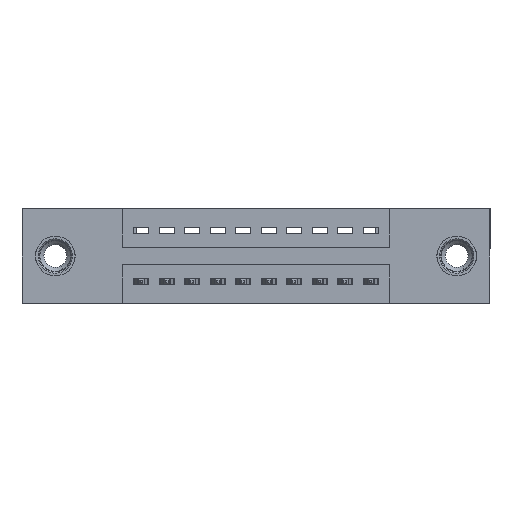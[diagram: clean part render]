
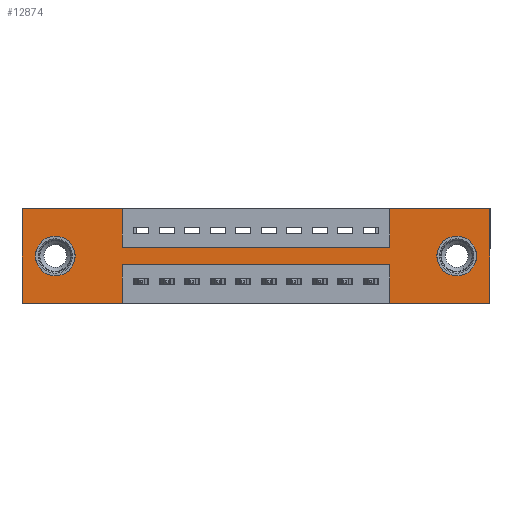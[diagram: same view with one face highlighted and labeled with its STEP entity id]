
A CAD part, front view. The second image highlights one B-rep face of the part: STEP entity #12874.
In plain terms, the highlighted planar face has unit normal (0, -1, 0).
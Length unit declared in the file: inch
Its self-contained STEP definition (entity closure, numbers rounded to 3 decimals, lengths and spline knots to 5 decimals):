
#21 = CARTESIAN_POINT ( 'NONE',  ( 0.3925, 0., -0.37 ) ) ;
#254 = EDGE_CURVE ( 'NONE', #4813, #13213, #10833, .T. ) ;
#297 = CARTESIAN_POINT ( 'NONE',  ( 1.835, 0., -0.37 ) ) ;
#329 = EDGE_CURVE ( 'NONE', #13062, #12910, #3905, .T. ) ;
#353 = CARTESIAN_POINT ( 'NONE',  ( 1.4425, 0., 0. ) ) ;
#485 = FACE_OUTER_BOUND ( 'NONE', #8280, .T. ) ;
#573 = ORIENTED_EDGE ( 'NONE', *, *, #7444, .F. ) ;
#635 = LINE ( 'NONE', #4767, #5573 ) ;
#639 = EDGE_LOOP ( 'NONE', ( #13489, #12977 ) ) ;
#645 = FACE_BOUND ( 'NONE', #639, .T. ) ;
#825 = LINE ( 'NONE', #1271, #7151 ) ;
#924 = VECTOR ( 'NONE', #7887, 39.37008 ) ;
#990 = EDGE_CURVE ( 'NONE', #11762, #13683, #10135, .T. ) ;
#1068 = DIRECTION ( 'NONE',  ( 0., 0., 1. ) ) ;
#1110 = VERTEX_POINT ( 'NONE', #7105 ) ;
#1271 = CARTESIAN_POINT ( 'NONE',  ( 0.3925, 0., 0. ) ) ;
#1292 = ORIENTED_EDGE ( 'NONE', *, *, #13262, .F. ) ;
#1466 = LINE ( 'NONE', #4617, #9600 ) ;
#1613 = CIRCLE ( 'NONE', #13138, 0.078 ) ;
#1667 = DIRECTION ( 'NONE',  ( 0., 1., 0. ) ) ;
#1796 = DIRECTION ( 'NONE',  ( 0., 0., -1. ) ) ;
#1991 = LINE ( 'NONE', #3376, #7304 ) ;
#2018 = EDGE_CURVE ( 'NONE', #13213, #4813, #1613, .T. ) ;
#2021 = DIRECTION ( 'NONE',  ( -1., 0., 0. ) ) ;
#2097 = EDGE_LOOP ( 'NONE', ( #10883, #4486 ) ) ;
#2165 = CARTESIAN_POINT ( 'NONE',  ( 1.4425, 0., -0.15 ) ) ;
#2184 = VECTOR ( 'NONE', #11891, 39.37008 ) ;
#2404 = DIRECTION ( 'NONE',  ( 0., 0., -1. ) ) ;
#2569 = ORIENTED_EDGE ( 'NONE', *, *, #990, .F. ) ;
#2615 = ORIENTED_EDGE ( 'NONE', *, *, #13657, .F. ) ;
#2635 = EDGE_CURVE ( 'NONE', #13719, #9156, #3951, .T. ) ;
#2650 = ORIENTED_EDGE ( 'NONE', *, *, #5373, .F. ) ;
#2685 = VECTOR ( 'NONE', #10183, 39.37008 ) ;
#2769 = CARTESIAN_POINT ( 'NONE',  ( 0., 0., -0.37 ) ) ;
#3183 = ORIENTED_EDGE ( 'NONE', *, *, #4160, .F. ) ;
#3193 = CARTESIAN_POINT ( 'NONE',  ( 0.13, 0., -0.185 ) ) ;
#3329 = EDGE_CURVE ( 'NONE', #9156, #13719, #5635, .T. ) ;
#3376 = CARTESIAN_POINT ( 'NONE',  ( 0.3925, 0., -0.22 ) ) ;
#3476 = DIRECTION ( 'NONE',  ( 1., 0., 0. ) ) ;
#3497 = ORIENTED_EDGE ( 'NONE', *, *, #5838, .F. ) ;
#3560 = VECTOR ( 'NONE', #13207, 39.37008 ) ;
#3574 = PLANE ( 'NONE',  #7757 ) ;
#3626 = VERTEX_POINT ( 'NONE', #6912 ) ;
#3708 = CARTESIAN_POINT ( 'NONE',  ( 0., 0., 0. ) ) ;
#3786 = DIRECTION ( 'NONE',  ( 0., 0., 1. ) ) ;
#3905 = LINE ( 'NONE', #11838, #9671 ) ;
#3951 = CIRCLE ( 'NONE', #12608, 0.078 ) ;
#3990 = CARTESIAN_POINT ( 'NONE',  ( 1.705, 0., -0.185 ) ) ;
#4160 = EDGE_CURVE ( 'NONE', #10180, #9082, #10006, .T. ) ;
#4393 = VERTEX_POINT ( 'NONE', #11444 ) ;
#4460 = ORIENTED_EDGE ( 'NONE', *, *, #5214, .F. ) ;
#4486 = ORIENTED_EDGE ( 'NONE', *, *, #2018, .T. ) ;
#4598 = CARTESIAN_POINT ( 'NONE',  ( 0.3925, 0., -0.37 ) ) ;
#4617 = CARTESIAN_POINT ( 'NONE',  ( 0., 0., 0. ) ) ;
#4648 = AXIS2_PLACEMENT_3D ( 'NONE', #3990, #7301, #10411 ) ;
#4767 = CARTESIAN_POINT ( 'NONE',  ( 0.3925, 0., -0.15 ) ) ;
#4813 = VERTEX_POINT ( 'NONE', #13123 ) ;
#5049 = DIRECTION ( 'NONE',  ( 0., 0., -1. ) ) ;
#5167 = CARTESIAN_POINT ( 'NONE',  ( 0., 0., 0. ) ) ;
#5214 = EDGE_CURVE ( 'NONE', #1110, #4393, #5613, .T. ) ;
#5373 = EDGE_CURVE ( 'NONE', #8755, #3626, #825, .T. ) ;
#5573 = VECTOR ( 'NONE', #11358, 39.37008 ) ;
#5613 = LINE ( 'NONE', #5167, #3560 ) ;
#5635 = CIRCLE ( 'NONE', #4648, 0.078 ) ;
#5718 = DIRECTION ( 'NONE',  ( 0., -1., 0. ) ) ;
#5820 = AXIS2_PLACEMENT_3D ( 'NONE', #11392, #1667, #3786 ) ;
#5838 = EDGE_CURVE ( 'NONE', #9082, #1110, #10962, .T. ) ;
#6062 = VECTOR ( 'NONE', #2021, 39.37008 ) ;
#6241 = CARTESIAN_POINT ( 'NONE',  ( 1.705, 0., -0.107 ) ) ;
#6496 = DIRECTION ( 'NONE',  ( 0., 1., 0. ) ) ;
#6734 = CARTESIAN_POINT ( 'NONE',  ( 1.705, 0., -0.185 ) ) ;
#6805 = ORIENTED_EDGE ( 'NONE', *, *, #8927, .F. ) ;
#6809 = EDGE_CURVE ( 'NONE', #9452, #13062, #1466, .T. ) ;
#6892 = CARTESIAN_POINT ( 'NONE',  ( 1.705, 0., -0.263 ) ) ;
#6912 = CARTESIAN_POINT ( 'NONE',  ( 0.3925, 0., -0.15 ) ) ;
#7029 = DIRECTION ( 'NONE',  ( 0., 0., -1. ) ) ;
#7105 = CARTESIAN_POINT ( 'NONE',  ( 0., 0., -0.37 ) ) ;
#7151 = VECTOR ( 'NONE', #1796, 39.37008 ) ;
#7256 = CARTESIAN_POINT ( 'NONE',  ( 0.3925, 0., -0.22 ) ) ;
#7301 = DIRECTION ( 'NONE',  ( 0., 1., 0. ) ) ;
#7304 = VECTOR ( 'NONE', #12032, 39.37008 ) ;
#7444 = EDGE_CURVE ( 'NONE', #12161, #9452, #13274, .T. ) ;
#7558 = DIRECTION ( 'NONE',  ( 0., 0., 1. ) ) ;
#7757 = AXIS2_PLACEMENT_3D ( 'NONE', #7921, #5718, #13106 ) ;
#7887 = DIRECTION ( 'NONE',  ( 0., 0., 1. ) ) ;
#7921 = CARTESIAN_POINT ( 'NONE',  ( 0., 0., -0.37 ) ) ;
#8280 = EDGE_LOOP ( 'NONE', ( #3183, #1292, #2569, #6805, #12929, #10810, #573, #2615, #2650, #13267, #4460, #3497 ) ) ;
#8353 = CARTESIAN_POINT ( 'NONE',  ( 1.4425, 0., 0. ) ) ;
#8510 = CARTESIAN_POINT ( 'NONE',  ( 0.13, 0., -0.263 ) ) ;
#8755 = VERTEX_POINT ( 'NONE', #13372 ) ;
#8927 = EDGE_CURVE ( 'NONE', #12910, #11762, #11769, .T. ) ;
#8985 = FACE_BOUND ( 'NONE', #2097, .T. ) ;
#9082 = VERTEX_POINT ( 'NONE', #21 ) ;
#9156 = VERTEX_POINT ( 'NONE', #6892 ) ;
#9215 = VECTOR ( 'NONE', #2404, 39.37008 ) ;
#9452 = VERTEX_POINT ( 'NONE', #8353 ) ;
#9600 = VECTOR ( 'NONE', #3476, 39.37008 ) ;
#9671 = VECTOR ( 'NONE', #5049, 39.37008 ) ;
#10006 = LINE ( 'NONE', #4598, #9215 ) ;
#10135 = LINE ( 'NONE', #11844, #13017 ) ;
#10180 = VERTEX_POINT ( 'NONE', #7256 ) ;
#10183 = DIRECTION ( 'NONE',  ( 1., 0., 0. ) ) ;
#10411 = DIRECTION ( 'NONE',  ( 0., 0., -1. ) ) ;
#10810 = ORIENTED_EDGE ( 'NONE', *, *, #6809, .F. ) ;
#10833 = CIRCLE ( 'NONE', #5820, 0.078 ) ;
#10883 = ORIENTED_EDGE ( 'NONE', *, *, #254, .T. ) ;
#10906 = CARTESIAN_POINT ( 'NONE',  ( 1.4425, 0., -0.37 ) ) ;
#10962 = LINE ( 'NONE', #2769, #2184 ) ;
#11271 = CARTESIAN_POINT ( 'NONE',  ( 1.835, 0., 0. ) ) ;
#11358 = DIRECTION ( 'NONE',  ( 1., 0., 0. ) ) ;
#11392 = CARTESIAN_POINT ( 'NONE',  ( 0.13, 0., -0.185 ) ) ;
#11444 = CARTESIAN_POINT ( 'NONE',  ( 0., 0., 0. ) ) ;
#11762 = VERTEX_POINT ( 'NONE', #10906 ) ;
#11769 = LINE ( 'NONE', #12950, #6062 ) ;
#11838 = CARTESIAN_POINT ( 'NONE',  ( 1.835, 0., 0. ) ) ;
#11844 = CARTESIAN_POINT ( 'NONE',  ( 1.4425, 0., -0.37 ) ) ;
#11891 = DIRECTION ( 'NONE',  ( -1., 0., 0. ) ) ;
#12032 = DIRECTION ( 'NONE',  ( -1., 0., 0. ) ) ;
#12161 = VERTEX_POINT ( 'NONE', #2165 ) ;
#12323 = DIRECTION ( 'NONE',  ( 0., 1., 0. ) ) ;
#12608 = AXIS2_PLACEMENT_3D ( 'NONE', #6734, #12323, #7029 ) ;
#12673 = LINE ( 'NONE', #3708, #2685 ) ;
#12874 = ADVANCED_FACE ( 'NONE', ( #645, #8985, #485 ), #3574, .T. ) ;
#12910 = VERTEX_POINT ( 'NONE', #297 ) ;
#12929 = ORIENTED_EDGE ( 'NONE', *, *, #329, .F. ) ;
#12950 = CARTESIAN_POINT ( 'NONE',  ( 0., 0., -0.37 ) ) ;
#12977 = ORIENTED_EDGE ( 'NONE', *, *, #3329, .T. ) ;
#13001 = EDGE_CURVE ( 'NONE', #4393, #8755, #12673, .T. ) ;
#13017 = VECTOR ( 'NONE', #7558, 39.37008 ) ;
#13062 = VERTEX_POINT ( 'NONE', #11271 ) ;
#13106 = DIRECTION ( 'NONE',  ( 0., 0., -1. ) ) ;
#13123 = CARTESIAN_POINT ( 'NONE',  ( 0.13, 0., -0.107 ) ) ;
#13138 = AXIS2_PLACEMENT_3D ( 'NONE', #3193, #6496, #1068 ) ;
#13207 = DIRECTION ( 'NONE',  ( 0., 0., 1. ) ) ;
#13213 = VERTEX_POINT ( 'NONE', #8510 ) ;
#13262 = EDGE_CURVE ( 'NONE', #13683, #10180, #1991, .T. ) ;
#13267 = ORIENTED_EDGE ( 'NONE', *, *, #13001, .F. ) ;
#13274 = LINE ( 'NONE', #353, #924 ) ;
#13372 = CARTESIAN_POINT ( 'NONE',  ( 0.3925, 0., 0. ) ) ;
#13489 = ORIENTED_EDGE ( 'NONE', *, *, #2635, .T. ) ;
#13627 = CARTESIAN_POINT ( 'NONE',  ( 1.4425, 0., -0.22 ) ) ;
#13657 = EDGE_CURVE ( 'NONE', #3626, #12161, #635, .T. ) ;
#13683 = VERTEX_POINT ( 'NONE', #13627 ) ;
#13719 = VERTEX_POINT ( 'NONE', #6241 ) ;
